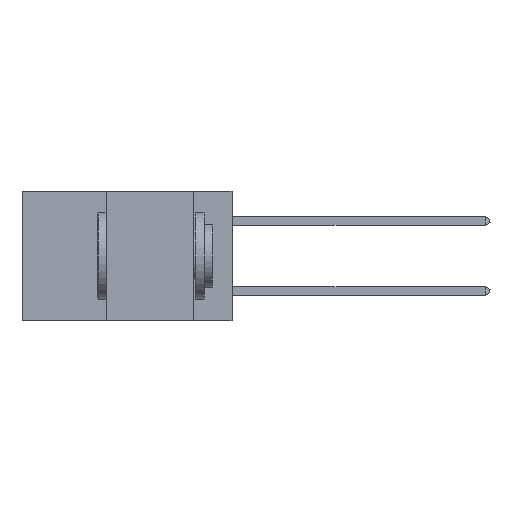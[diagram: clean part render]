
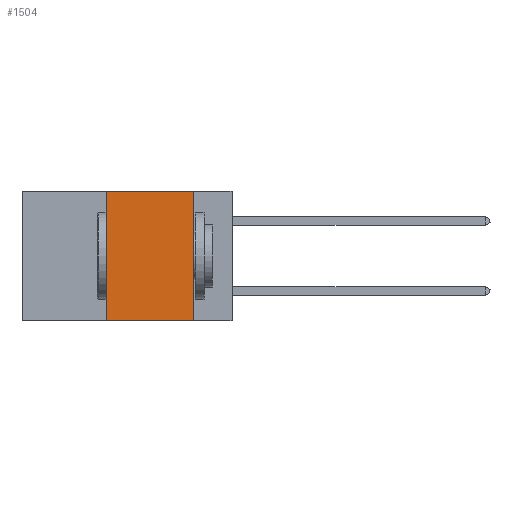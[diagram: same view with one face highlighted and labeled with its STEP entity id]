
A CAD part, left-side view. The second image highlights one B-rep face of the part: STEP entity #1504.
In plain terms, the highlighted planar face has unit normal (-1, 0, 0).
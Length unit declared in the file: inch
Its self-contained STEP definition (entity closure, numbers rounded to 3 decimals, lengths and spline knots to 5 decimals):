
#209 = EDGE_CURVE ( 'NONE', #3081, #12894, #11251, .T. ) ;
#331 = ORIENTED_EDGE ( 'NONE', *, *, #761, .T. ) ;
#373 = LINE ( 'NONE', #1996, #8089 ) ;
#659 = VERTEX_POINT ( 'NONE', #12878 ) ;
#761 = EDGE_CURVE ( 'NONE', #659, #12894, #7946, .T. ) ;
#1504 = ADVANCED_FACE ( 'NONE', ( #10342 ), #12984, .F. ) ;
#1671 = DIRECTION ( 'NONE',  ( 0., 0., -1. ) ) ;
#1996 = CARTESIAN_POINT ( 'NONE',  ( 0., 0.36, 0. ) ) ;
#2558 = VERTEX_POINT ( 'NONE', #7120 ) ;
#2739 = EDGE_LOOP ( 'NONE', ( #11802, #14696, #9234, #331 ) ) ;
#2924 = DIRECTION ( 'NONE',  ( 0., -1., 0. ) ) ;
#3064 = DIRECTION ( 'NONE',  ( 0., -1., 0. ) ) ;
#3081 = VERTEX_POINT ( 'NONE', #6249 ) ;
#3103 = CARTESIAN_POINT ( 'NONE',  ( 0., 0.6, 0. ) ) ;
#3214 = DIRECTION ( 'NONE',  ( 0., 0., 1. ) ) ;
#4025 = EDGE_CURVE ( 'NONE', #2558, #3081, #13022, .T. ) ;
#4893 = AXIS2_PLACEMENT_3D ( 'NONE', #7022, #14474, #1671 ) ;
#6249 = CARTESIAN_POINT ( 'NONE',  ( 0., 0.11, 0. ) ) ;
#7022 = CARTESIAN_POINT ( 'NONE',  ( 0., 0.6, 0. ) ) ;
#7120 = CARTESIAN_POINT ( 'NONE',  ( 0., 0.36, 0. ) ) ;
#7590 = VECTOR ( 'NONE', #2924, 39.37008 ) ;
#7946 = LINE ( 'NONE', #8118, #7590 ) ;
#7986 = DIRECTION ( 'NONE',  ( 0., 0., -1. ) ) ;
#8089 = VECTOR ( 'NONE', #3214, 39.37008 ) ;
#8118 = CARTESIAN_POINT ( 'NONE',  ( 0., 0.6, -0.37 ) ) ;
#9234 = ORIENTED_EDGE ( 'NONE', *, *, #12089, .F. ) ;
#10109 = VECTOR ( 'NONE', #3064, 39.37008 ) ;
#10342 = FACE_OUTER_BOUND ( 'NONE', #2739, .T. ) ;
#11251 = LINE ( 'NONE', #12382, #11942 ) ;
#11802 = ORIENTED_EDGE ( 'NONE', *, *, #209, .F. ) ;
#11942 = VECTOR ( 'NONE', #7986, 39.37008 ) ;
#12089 = EDGE_CURVE ( 'NONE', #659, #2558, #373, .T. ) ;
#12382 = CARTESIAN_POINT ( 'NONE',  ( 0., 0.11, 0. ) ) ;
#12878 = CARTESIAN_POINT ( 'NONE',  ( 0., 0.36, -0.37 ) ) ;
#12894 = VERTEX_POINT ( 'NONE', #13579 ) ;
#12984 = PLANE ( 'NONE',  #4893 ) ;
#13022 = LINE ( 'NONE', #3103, #10109 ) ;
#13579 = CARTESIAN_POINT ( 'NONE',  ( 0., 0.11, -0.37 ) ) ;
#14474 = DIRECTION ( 'NONE',  ( 1., 0., 0. ) ) ;
#14696 = ORIENTED_EDGE ( 'NONE', *, *, #4025, .F. ) ;
